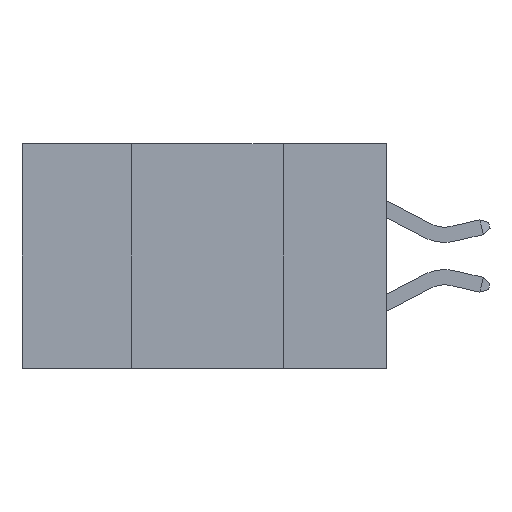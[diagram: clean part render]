
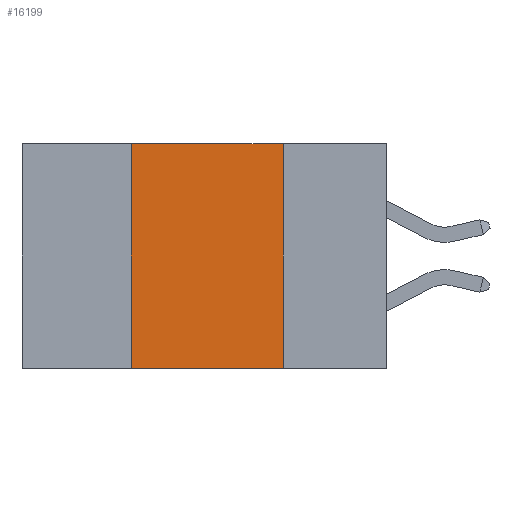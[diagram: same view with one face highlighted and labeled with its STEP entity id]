
A CAD part, left-side view. The second image highlights one B-rep face of the part: STEP entity #16199.
In plain terms, the highlighted planar face has unit normal (-1, 0, 0).
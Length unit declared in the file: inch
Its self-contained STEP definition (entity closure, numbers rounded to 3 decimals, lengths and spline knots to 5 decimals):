
#1335 = DIRECTION ( 'NONE',  ( 0., 0., -1. ) ) ;
#2427 = DIRECTION ( 'NONE',  ( 1., 0., 0. ) ) ;
#3160 = VERTEX_POINT ( 'NONE', #20583 ) ;
#4369 = DIRECTION ( 'NONE',  ( 0., 0., -1. ) ) ;
#4717 = PLANE ( 'NONE',  #11119 ) ;
#4747 = LINE ( 'NONE', #8976, #20347 ) ;
#4894 = LINE ( 'NONE', #17762, #12565 ) ;
#5489 = CARTESIAN_POINT ( 'NONE',  ( 0., 0.6, -0.37 ) ) ;
#5563 = DIRECTION ( 'NONE',  ( 0., 0., 1. ) ) ;
#6762 = ORIENTED_EDGE ( 'NONE', *, *, #7083, .F. ) ;
#7083 = EDGE_CURVE ( 'NONE', #17276, #3160, #4894, .T. ) ;
#7541 = LINE ( 'NONE', #5489, #18026 ) ;
#8976 = CARTESIAN_POINT ( 'NONE',  ( 0., 0.17, 0. ) ) ;
#9358 = FACE_OUTER_BOUND ( 'NONE', #22144, .T. ) ;
#9858 = VECTOR ( 'NONE', #19059, 39.37008 ) ;
#10995 = CARTESIAN_POINT ( 'NONE',  ( 0., 0.6, 0. ) ) ;
#11119 = AXIS2_PLACEMENT_3D ( 'NONE', #12591, #2427, #4369 ) ;
#11205 = ORIENTED_EDGE ( 'NONE', *, *, #21157, .F. ) ;
#12565 = VECTOR ( 'NONE', #5563, 39.37008 ) ;
#12591 = CARTESIAN_POINT ( 'NONE',  ( 0., 0.6, 0. ) ) ;
#13119 = ORIENTED_EDGE ( 'NONE', *, *, #17782, .T. ) ;
#15248 = VERTEX_POINT ( 'NONE', #26286 ) ;
#16199 = ADVANCED_FACE ( 'NONE', ( #9358 ), #4717, .F. ) ;
#17276 = VERTEX_POINT ( 'NONE', #18544 ) ;
#17762 = CARTESIAN_POINT ( 'NONE',  ( 0., 0.42, 0. ) ) ;
#17765 = EDGE_CURVE ( 'NONE', #22619, #15248, #4747, .T. ) ;
#17782 = EDGE_CURVE ( 'NONE', #17276, #15248, #7541, .T. ) ;
#17849 = DIRECTION ( 'NONE',  ( 0., -1., 0. ) ) ;
#18026 = VECTOR ( 'NONE', #17849, 39.37008 ) ;
#18544 = CARTESIAN_POINT ( 'NONE',  ( 0., 0.42, -0.37 ) ) ;
#19059 = DIRECTION ( 'NONE',  ( 0., -1., 0. ) ) ;
#20134 = ORIENTED_EDGE ( 'NONE', *, *, #17765, .F. ) ;
#20347 = VECTOR ( 'NONE', #1335, 39.37008 ) ;
#20583 = CARTESIAN_POINT ( 'NONE',  ( 0., 0.42, 0. ) ) ;
#21157 = EDGE_CURVE ( 'NONE', #3160, #22619, #21328, .T. ) ;
#21328 = LINE ( 'NONE', #10995, #9858 ) ;
#22144 = EDGE_LOOP ( 'NONE', ( #20134, #11205, #6762, #13119 ) ) ;
#22619 = VERTEX_POINT ( 'NONE', #23581 ) ;
#23581 = CARTESIAN_POINT ( 'NONE',  ( 0., 0.17, 0. ) ) ;
#26286 = CARTESIAN_POINT ( 'NONE',  ( 0., 0.17, -0.37 ) ) ;
